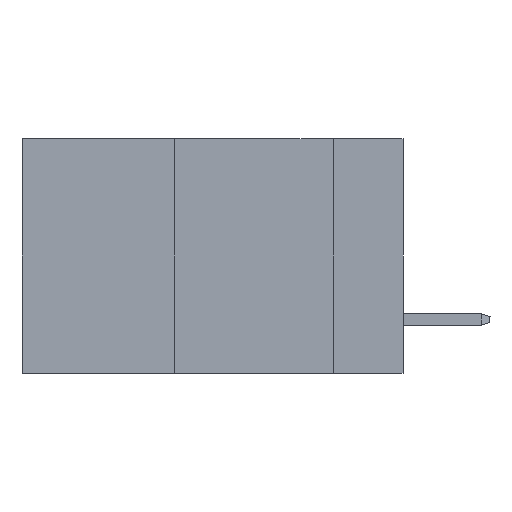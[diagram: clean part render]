
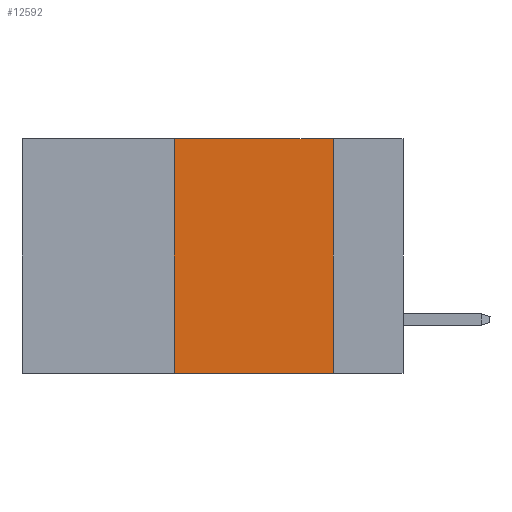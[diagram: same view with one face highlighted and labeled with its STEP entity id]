
A CAD part, left-side view. The second image highlights one B-rep face of the part: STEP entity #12592.
In plain terms, the highlighted planar face has unit normal (-1, 0, 0).
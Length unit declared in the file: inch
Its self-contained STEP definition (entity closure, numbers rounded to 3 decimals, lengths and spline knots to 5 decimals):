
#1003 = VERTEX_POINT ( 'NONE', #13345 ) ;
#1007 = VECTOR ( 'NONE', #1277, 39.37008 ) ;
#1058 = CARTESIAN_POINT ( 'NONE',  ( 0., 0.36, 0. ) ) ;
#1277 = DIRECTION ( 'NONE',  ( 0., -1., 0. ) ) ;
#2328 = LINE ( 'NONE', #9972, #7691 ) ;
#2406 = EDGE_CURVE ( 'NONE', #1003, #4070, #2328, .T. ) ;
#2458 = FACE_OUTER_BOUND ( 'NONE', #13436, .T. ) ;
#2480 = VECTOR ( 'NONE', #4016, 39.37008 ) ;
#2670 = DIRECTION ( 'NONE',  ( 0., 0., -1. ) ) ;
#3383 = ORIENTED_EDGE ( 'NONE', *, *, #12473, .F. ) ;
#3847 = CARTESIAN_POINT ( 'NONE',  ( 0., 0.11, -0.37 ) ) ;
#4016 = DIRECTION ( 'NONE',  ( 0., 0., 1. ) ) ;
#4070 = VERTEX_POINT ( 'NONE', #3847 ) ;
#4179 = CARTESIAN_POINT ( 'NONE',  ( 0., 0.11, 0. ) ) ;
#4624 = PLANE ( 'NONE',  #11433 ) ;
#4768 = EDGE_CURVE ( 'NONE', #5118, #7669, #5545, .T. ) ;
#5118 = VERTEX_POINT ( 'NONE', #1058 ) ;
#5308 = ORIENTED_EDGE ( 'NONE', *, *, #12062, .F. ) ;
#5545 = LINE ( 'NONE', #13061, #1007 ) ;
#6179 = DIRECTION ( 'NONE',  ( 0., 0., -1. ) ) ;
#6294 = LINE ( 'NONE', #7420, #2480 ) ;
#7420 = CARTESIAN_POINT ( 'NONE',  ( 0., 0.36, 0. ) ) ;
#7669 = VERTEX_POINT ( 'NONE', #9813 ) ;
#7691 = VECTOR ( 'NONE', #12073, 39.37008 ) ;
#7983 = DIRECTION ( 'NONE',  ( 1., 0., 0. ) ) ;
#9813 = CARTESIAN_POINT ( 'NONE',  ( 0., 0.11, 0. ) ) ;
#9972 = CARTESIAN_POINT ( 'NONE',  ( 0., 0.6, -0.37 ) ) ;
#10000 = ORIENTED_EDGE ( 'NONE', *, *, #2406, .T. ) ;
#10614 = LINE ( 'NONE', #4179, #12793 ) ;
#11010 = CARTESIAN_POINT ( 'NONE',  ( 0., 0.6, 0. ) ) ;
#11433 = AXIS2_PLACEMENT_3D ( 'NONE', #11010, #7983, #2670 ) ;
#11829 = ORIENTED_EDGE ( 'NONE', *, *, #4768, .F. ) ;
#12062 = EDGE_CURVE ( 'NONE', #1003, #5118, #6294, .T. ) ;
#12073 = DIRECTION ( 'NONE',  ( 0., -1., 0. ) ) ;
#12473 = EDGE_CURVE ( 'NONE', #7669, #4070, #10614, .T. ) ;
#12592 = ADVANCED_FACE ( 'NONE', ( #2458 ), #4624, .F. ) ;
#12793 = VECTOR ( 'NONE', #6179, 39.37008 ) ;
#13061 = CARTESIAN_POINT ( 'NONE',  ( 0., 0.6, 0. ) ) ;
#13345 = CARTESIAN_POINT ( 'NONE',  ( 0., 0.36, -0.37 ) ) ;
#13436 = EDGE_LOOP ( 'NONE', ( #3383, #11829, #5308, #10000 ) ) ;
